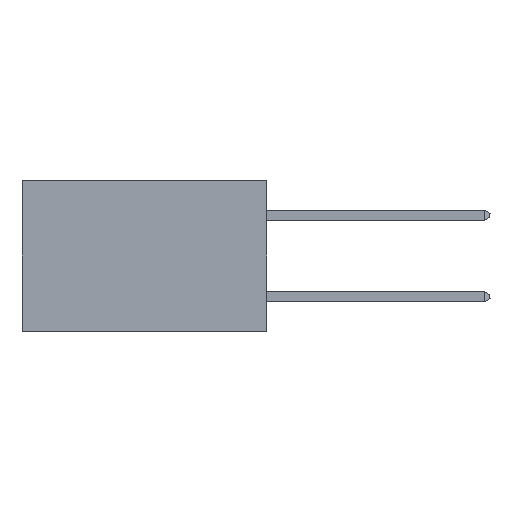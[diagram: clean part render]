
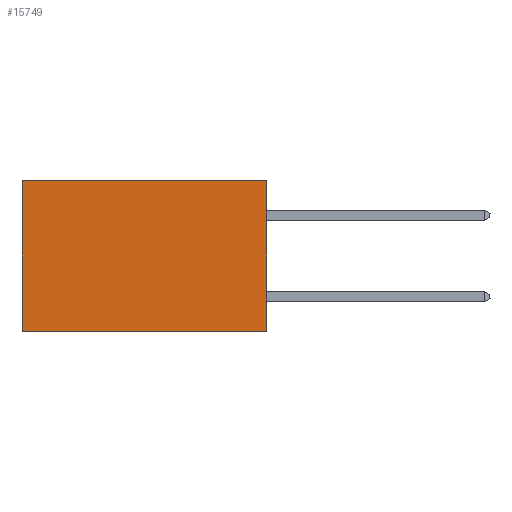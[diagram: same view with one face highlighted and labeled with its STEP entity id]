
A CAD part, left-side view. The second image highlights one B-rep face of the part: STEP entity #15749.
In plain terms, the highlighted planar face has unit normal (-1, 0, 0).
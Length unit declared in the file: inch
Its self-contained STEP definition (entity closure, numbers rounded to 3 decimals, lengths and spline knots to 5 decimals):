
#1137 = DIRECTION ( 'NONE',  ( 1., 0., 0. ) ) ;
#1673 = EDGE_CURVE ( 'NONE', #25676, #33164, #24444, .T. ) ;
#2868 = AXIS2_PLACEMENT_3D ( 'NONE', #9884, #1137, #21399 ) ;
#5187 = ORIENTED_EDGE ( 'NONE', *, *, #5524, .F. ) ;
#5346 = CARTESIAN_POINT ( 'NONE',  ( 0.2875, 0., 0. ) ) ;
#5524 = EDGE_CURVE ( 'NONE', #8569, #27455, #35360, .T. ) ;
#5640 = ORIENTED_EDGE ( 'NONE', *, *, #19677, .T. ) ;
#7414 = CARTESIAN_POINT ( 'NONE',  ( 0.2875, 0., -0.37 ) ) ;
#8569 = VERTEX_POINT ( 'NONE', #5346 ) ;
#9884 = CARTESIAN_POINT ( 'NONE',  ( 0.2875, 0., 0. ) ) ;
#10519 = DIRECTION ( 'NONE',  ( 0., 0., -1. ) ) ;
#10675 = FACE_OUTER_BOUND ( 'NONE', #35757, .T. ) ;
#15749 = ADVANCED_FACE ( 'NONE', ( #10675 ), #18566, .F. ) ;
#16892 = VECTOR ( 'NONE', #10519, 39.37008 ) ;
#18566 = PLANE ( 'NONE',  #2868 ) ;
#19065 = ORIENTED_EDGE ( 'NONE', *, *, #1673, .T. ) ;
#19677 = EDGE_CURVE ( 'NONE', #8569, #25676, #33150, .T. ) ;
#20728 = CARTESIAN_POINT ( 'NONE',  ( 0.2875, 0., -0.37 ) ) ;
#20802 = CARTESIAN_POINT ( 'NONE',  ( 0.2875, 0., 0. ) ) ;
#21399 = DIRECTION ( 'NONE',  ( 0., 0., -1. ) ) ;
#24444 = LINE ( 'NONE', #33384, #16892 ) ;
#25415 = CARTESIAN_POINT ( 'NONE',  ( 0.2875, 0., 0. ) ) ;
#25587 = VECTOR ( 'NONE', #36844, 39.37008 ) ;
#25676 = VERTEX_POINT ( 'NONE', #36248 ) ;
#27455 = VERTEX_POINT ( 'NONE', #7414 ) ;
#29371 = LINE ( 'NONE', #20728, #36877 ) ;
#32239 = DIRECTION ( 'NONE',  ( 0., 1., 0. ) ) ;
#33150 = LINE ( 'NONE', #25415, #25587 ) ;
#33164 = VERTEX_POINT ( 'NONE', #34552 ) ;
#33384 = CARTESIAN_POINT ( 'NONE',  ( 0.2875, 0.6, 0. ) ) ;
#33595 = VECTOR ( 'NONE', #35028, 39.37008 ) ;
#34552 = CARTESIAN_POINT ( 'NONE',  ( 0.2875, 0.6, -0.37 ) ) ;
#35028 = DIRECTION ( 'NONE',  ( 0., 0., -1. ) ) ;
#35360 = LINE ( 'NONE', #20802, #33595 ) ;
#35726 = EDGE_CURVE ( 'NONE', #27455, #33164, #29371, .T. ) ;
#35757 = EDGE_LOOP ( 'NONE', ( #19065, #35825, #5187, #5640 ) ) ;
#35825 = ORIENTED_EDGE ( 'NONE', *, *, #35726, .F. ) ;
#36248 = CARTESIAN_POINT ( 'NONE',  ( 0.2875, 0.6, 0. ) ) ;
#36844 = DIRECTION ( 'NONE',  ( 0., 1., 0. ) ) ;
#36877 = VECTOR ( 'NONE', #32239, 39.37008 ) ;
